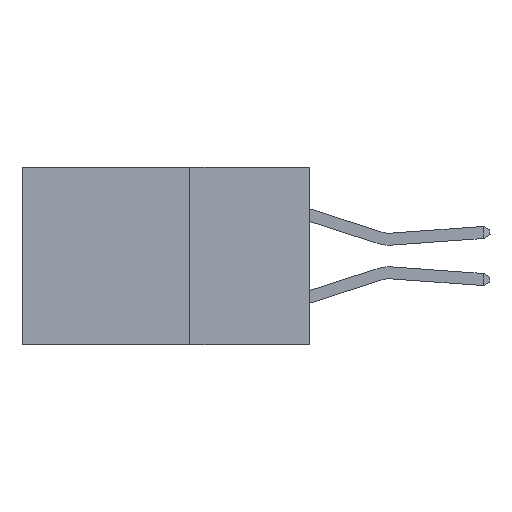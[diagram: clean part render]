
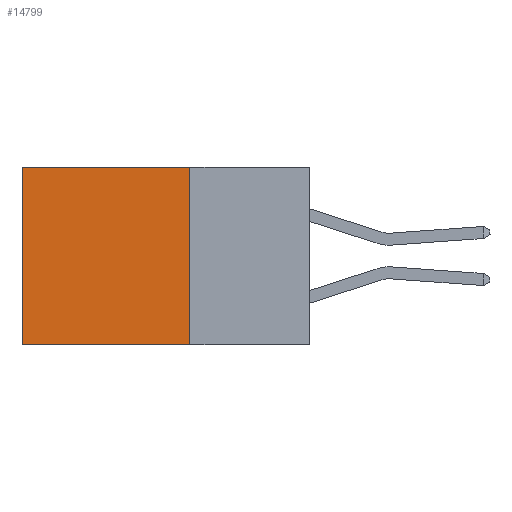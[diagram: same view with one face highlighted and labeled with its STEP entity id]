
A CAD part, left-side view. The second image highlights one B-rep face of the part: STEP entity #14799.
In plain terms, the highlighted planar face has unit normal (-1, 0, 0).
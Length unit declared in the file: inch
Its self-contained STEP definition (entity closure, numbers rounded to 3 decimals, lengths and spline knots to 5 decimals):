
#373 = VERTEX_POINT ( 'NONE', #12512 ) ;
#625 = VECTOR ( 'NONE', #4895, 39.37008 ) ;
#851 = LINE ( 'NONE', #14930, #10387 ) ;
#914 = ORIENTED_EDGE ( 'NONE', *, *, #14718, .T. ) ;
#944 = DIRECTION ( 'NONE',  ( 0., 0., -1. ) ) ;
#2092 = LINE ( 'NONE', #7407, #8576 ) ;
#3058 = EDGE_LOOP ( 'NONE', ( #914, #15033, #7259, #5174 ) ) ;
#4887 = VERTEX_POINT ( 'NONE', #11820 ) ;
#4895 = DIRECTION ( 'NONE',  ( 0., 1., 0. ) ) ;
#4919 = LINE ( 'NONE', #5031, #625 ) ;
#5031 = CARTESIAN_POINT ( 'NONE',  ( 0.2615, 0.25, -0.37 ) ) ;
#5174 = ORIENTED_EDGE ( 'NONE', *, *, #15238, .T. ) ;
#5424 = VERTEX_POINT ( 'NONE', #7923 ) ;
#5848 = EDGE_CURVE ( 'NONE', #15185, #5424, #4919, .T. ) ;
#7259 = ORIENTED_EDGE ( 'NONE', *, *, #14695, .F. ) ;
#7407 = CARTESIAN_POINT ( 'NONE',  ( 0.2615, 0.25, -0.37 ) ) ;
#7741 = DIRECTION ( 'NONE',  ( 0., 0., -1. ) ) ;
#7923 = CARTESIAN_POINT ( 'NONE',  ( 0.2615, 0.6, -0.37 ) ) ;
#8576 = VECTOR ( 'NONE', #14998, 39.37008 ) ;
#8620 = DIRECTION ( 'NONE',  ( 0., 1., 0. ) ) ;
#8702 = CARTESIAN_POINT ( 'NONE',  ( 0.2615, 0.6, -0.37 ) ) ;
#10387 = VECTOR ( 'NONE', #8620, 39.37008 ) ;
#11603 = VECTOR ( 'NONE', #944, 39.37008 ) ;
#11820 = CARTESIAN_POINT ( 'NONE',  ( 0.2615, 0.6, 0. ) ) ;
#12512 = CARTESIAN_POINT ( 'NONE',  ( 0.2615, 0.25, 0. ) ) ;
#12821 = CARTESIAN_POINT ( 'NONE',  ( 0.2615, 0.25, -0.37 ) ) ;
#13521 = CARTESIAN_POINT ( 'NONE',  ( 0.2615, 0.25, -0.37 ) ) ;
#13745 = FACE_OUTER_BOUND ( 'NONE', #3058, .T. ) ;
#14084 = PLANE ( 'NONE',  #15512 ) ;
#14695 = EDGE_CURVE ( 'NONE', #373, #15185, #2092, .T. ) ;
#14718 = EDGE_CURVE ( 'NONE', #4887, #5424, #14912, .T. ) ;
#14799 = ADVANCED_FACE ( 'NONE', ( #13745 ), #14084, .F. ) ;
#14912 = LINE ( 'NONE', #8702, #11603 ) ;
#14930 = CARTESIAN_POINT ( 'NONE',  ( 0.2615, 0.25, 0. ) ) ;
#14998 = DIRECTION ( 'NONE',  ( 0., 0., -1. ) ) ;
#15033 = ORIENTED_EDGE ( 'NONE', *, *, #5848, .F. ) ;
#15185 = VERTEX_POINT ( 'NONE', #13521 ) ;
#15238 = EDGE_CURVE ( 'NONE', #373, #4887, #851, .T. ) ;
#15309 = DIRECTION ( 'NONE',  ( 1., 0., 0. ) ) ;
#15512 = AXIS2_PLACEMENT_3D ( 'NONE', #12821, #15309, #7741 ) ;
